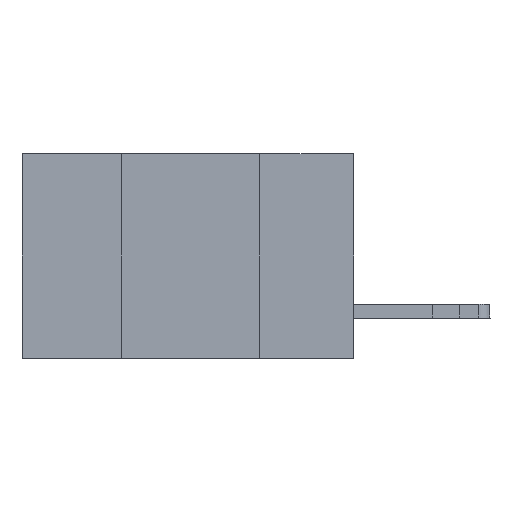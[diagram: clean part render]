
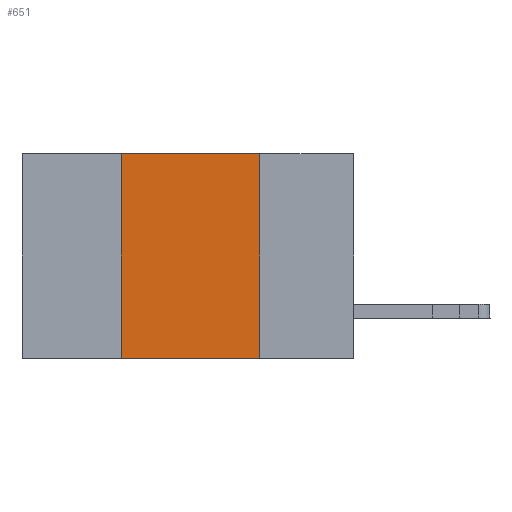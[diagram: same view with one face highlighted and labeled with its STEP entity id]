
A CAD part, left-side view. The second image highlights one B-rep face of the part: STEP entity #651.
In plain terms, the highlighted planar face has unit normal (-1, 0, 0).
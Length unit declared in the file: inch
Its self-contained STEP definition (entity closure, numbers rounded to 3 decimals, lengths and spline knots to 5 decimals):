
#651 = ADVANCED_FACE ( 'NONE', ( #27917 ), #7830, .F. ) ;
#673 = VERTEX_POINT ( 'NONE', #26577 ) ;
#1040 = AXIS2_PLACEMENT_3D ( 'NONE', #10206, #26482, #12570 ) ;
#3441 = CARTESIAN_POINT ( 'NONE',  ( 0., 0.6, -0.37 ) ) ;
#5060 = EDGE_CURVE ( 'NONE', #26286, #6807, #20005, .T. ) ;
#6544 = VECTOR ( 'NONE', #30187, 39.37008 ) ;
#6547 = VECTOR ( 'NONE', #29419, 39.37008 ) ;
#6807 = VERTEX_POINT ( 'NONE', #21892 ) ;
#7135 = CARTESIAN_POINT ( 'NONE',  ( 0., 0.17, 0. ) ) ;
#7231 = CARTESIAN_POINT ( 'NONE',  ( 0., 0.6, 0. ) ) ;
#7277 = LINE ( 'NONE', #17899, #6547 ) ;
#7551 = VECTOR ( 'NONE', #15225, 39.37008 ) ;
#7830 = PLANE ( 'NONE',  #1040 ) ;
#9387 = EDGE_CURVE ( 'NONE', #26286, #673, #25123, .T. ) ;
#9641 = ORIENTED_EDGE ( 'NONE', *, *, #23038, .F. ) ;
#9727 = ORIENTED_EDGE ( 'NONE', *, *, #27957, .F. ) ;
#10046 = ORIENTED_EDGE ( 'NONE', *, *, #9387, .F. ) ;
#10111 = ORIENTED_EDGE ( 'NONE', *, *, #5060, .T. ) ;
#10206 = CARTESIAN_POINT ( 'NONE',  ( 0., 0.6, 0. ) ) ;
#11040 = VECTOR ( 'NONE', #23555, 39.37008 ) ;
#12570 = DIRECTION ( 'NONE',  ( 0., 0., -1. ) ) ;
#15225 = DIRECTION ( 'NONE',  ( 0., -1., 0. ) ) ;
#17899 = CARTESIAN_POINT ( 'NONE',  ( 0., 0.17, 0. ) ) ;
#19399 = CARTESIAN_POINT ( 'NONE',  ( 0., 0.42, -0.37 ) ) ;
#20005 = LINE ( 'NONE', #3441, #7551 ) ;
#21892 = CARTESIAN_POINT ( 'NONE',  ( 0., 0.17, -0.37 ) ) ;
#23038 = EDGE_CURVE ( 'NONE', #29452, #6807, #7277, .T. ) ;
#23418 = LINE ( 'NONE', #7231, #11040 ) ;
#23555 = DIRECTION ( 'NONE',  ( 0., -1., 0. ) ) ;
#25123 = LINE ( 'NONE', #25432, #6544 ) ;
#25432 = CARTESIAN_POINT ( 'NONE',  ( 0., 0.42, 0. ) ) ;
#26286 = VERTEX_POINT ( 'NONE', #19399 ) ;
#26482 = DIRECTION ( 'NONE',  ( 1., 0., 0. ) ) ;
#26577 = CARTESIAN_POINT ( 'NONE',  ( 0., 0.42, 0. ) ) ;
#27627 = EDGE_LOOP ( 'NONE', ( #9641, #9727, #10046, #10111 ) ) ;
#27917 = FACE_OUTER_BOUND ( 'NONE', #27627, .T. ) ;
#27957 = EDGE_CURVE ( 'NONE', #673, #29452, #23418, .T. ) ;
#29419 = DIRECTION ( 'NONE',  ( 0., 0., -1. ) ) ;
#29452 = VERTEX_POINT ( 'NONE', #7135 ) ;
#30187 = DIRECTION ( 'NONE',  ( 0., 0., 1. ) ) ;
